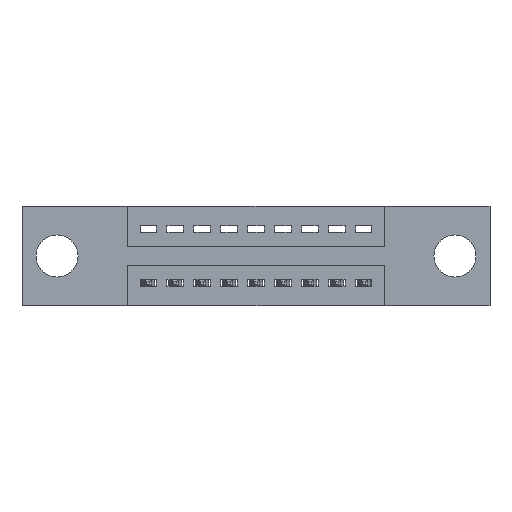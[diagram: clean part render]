
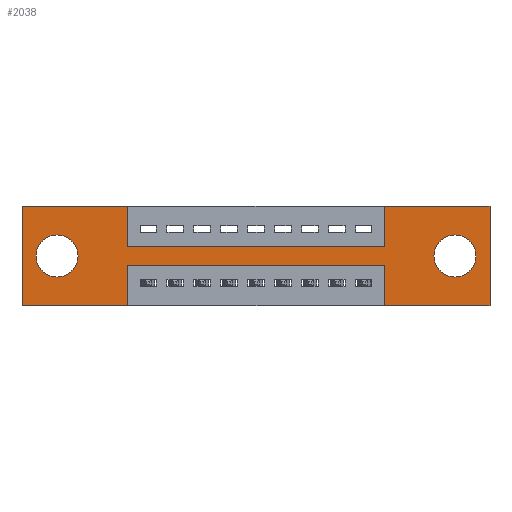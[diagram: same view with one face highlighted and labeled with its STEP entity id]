
A CAD part, front view. The second image highlights one B-rep face of the part: STEP entity #2038.
In plain terms, the highlighted planar face has unit normal (0, -1, 0).
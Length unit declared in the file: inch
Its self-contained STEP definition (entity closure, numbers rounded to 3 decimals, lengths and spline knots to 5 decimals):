
#24 = ORIENTED_EDGE ( 'NONE', *, *, #10581, .F. ) ;
#48 = DIRECTION ( 'NONE',  ( 0., 1., 0. ) ) ;
#113 = CARTESIAN_POINT ( 'NONE',  ( 0.13, 0., -0.185 ) ) ;
#126 = EDGE_LOOP ( 'NONE', ( #5890, #6085, #3829, #6019, #745, #6977, #2964, #5603, #10811, #10985, #5366, #24 ) ) ;
#154 = VECTOR ( 'NONE', #1543, 39.37008 ) ;
#226 = DIRECTION ( 'NONE',  ( 0., 1., 0. ) ) ;
#268 = CARTESIAN_POINT ( 'NONE',  ( 1.3425, 0., -0.15 ) ) ;
#337 = DIRECTION ( 'NONE',  ( 0., 0., -1. ) ) ;
#339 = CIRCLE ( 'NONE', #676, 0.078 ) ;
#390 = CARTESIAN_POINT ( 'NONE',  ( 0., 0., -0.37 ) ) ;
#392 = CIRCLE ( 'NONE', #1590, 0.078 ) ;
#396 = VERTEX_POINT ( 'NONE', #7209 ) ;
#422 = EDGE_CURVE ( 'NONE', #6330, #3517, #10646, .T. ) ;
#447 = CARTESIAN_POINT ( 'NONE',  ( 0.3925, 0., -0.22 ) ) ;
#501 = CARTESIAN_POINT ( 'NONE',  ( 1.605, 0., -0.263 ) ) ;
#584 = VECTOR ( 'NONE', #5580, 39.37008 ) ;
#661 = VECTOR ( 'NONE', #5711, 39.37008 ) ;
#672 = LINE ( 'NONE', #390, #9930 ) ;
#676 = AXIS2_PLACEMENT_3D ( 'NONE', #7832, #48, #2664 ) ;
#745 = ORIENTED_EDGE ( 'NONE', *, *, #4277, .F. ) ;
#799 = VERTEX_POINT ( 'NONE', #3179 ) ;
#807 = VERTEX_POINT ( 'NONE', #10939 ) ;
#849 = VECTOR ( 'NONE', #971, 39.37008 ) ;
#971 = DIRECTION ( 'NONE',  ( 0., 0., 1. ) ) ;
#1173 = CARTESIAN_POINT ( 'NONE',  ( 1.605, 0., -0.185 ) ) ;
#1176 = ORIENTED_EDGE ( 'NONE', *, *, #8504, .T. ) ;
#1543 = DIRECTION ( 'NONE',  ( -1., 0., 0. ) ) ;
#1576 = CARTESIAN_POINT ( 'NONE',  ( 1.735, 0., 0. ) ) ;
#1590 = AXIS2_PLACEMENT_3D ( 'NONE', #1173, #3766, #337 ) ;
#1688 = CARTESIAN_POINT ( 'NONE',  ( 0., 0., 0. ) ) ;
#1762 = CARTESIAN_POINT ( 'NONE',  ( 1.3425, 0., -0.22 ) ) ;
#2038 = ADVANCED_FACE ( 'NONE', ( #9285, #2340, #5317 ), #4694, .T. ) ;
#2233 = DIRECTION ( 'NONE',  ( 1., 0., 0. ) ) ;
#2272 = EDGE_CURVE ( 'NONE', #6221, #807, #6128, .T. ) ;
#2276 = DIRECTION ( 'NONE',  ( 0., 0., 1. ) ) ;
#2340 = FACE_BOUND ( 'NONE', #10150, .T. ) ;
#2423 = DIRECTION ( 'NONE',  ( 1., 0., 0. ) ) ;
#2607 = AXIS2_PLACEMENT_3D ( 'NONE', #6830, #6025, #8680 ) ;
#2634 = VERTEX_POINT ( 'NONE', #7970 ) ;
#2664 = DIRECTION ( 'NONE',  ( 0., 0., 1. ) ) ;
#2705 = CARTESIAN_POINT ( 'NONE',  ( 0.3925, 0., -0.22 ) ) ;
#2796 = CARTESIAN_POINT ( 'NONE',  ( 0., 0., 0. ) ) ;
#2964 = ORIENTED_EDGE ( 'NONE', *, *, #2272, .F. ) ;
#3005 = EDGE_CURVE ( 'NONE', #807, #10162, #8576, .T. ) ;
#3008 = DIRECTION ( 'NONE',  ( 0., 0., -1. ) ) ;
#3048 = LINE ( 'NONE', #2796, #8111 ) ;
#3080 = DIRECTION ( 'NONE',  ( 1., 0., 0. ) ) ;
#3179 = CARTESIAN_POINT ( 'NONE',  ( 0.13, 0., -0.107 ) ) ;
#3517 = VERTEX_POINT ( 'NONE', #1762 ) ;
#3636 = VERTEX_POINT ( 'NONE', #501 ) ;
#3766 = DIRECTION ( 'NONE',  ( 0., 1., 0. ) ) ;
#3829 = ORIENTED_EDGE ( 'NONE', *, *, #422, .F. ) ;
#3936 = VECTOR ( 'NONE', #2423, 39.37008 ) ;
#4048 = VERTEX_POINT ( 'NONE', #4956 ) ;
#4277 = EDGE_CURVE ( 'NONE', #10162, #396, #4987, .T. ) ;
#4488 = EDGE_CURVE ( 'NONE', #3636, #10643, #392, .T. ) ;
#4516 = DIRECTION ( 'NONE',  ( 0., 0., 1. ) ) ;
#4694 = PLANE ( 'NONE',  #7392 ) ;
#4696 = CARTESIAN_POINT ( 'NONE',  ( 1.605, 0., -0.107 ) ) ;
#4730 = EDGE_CURVE ( 'NONE', #10643, #3636, #4827, .T. ) ;
#4827 = CIRCLE ( 'NONE', #2607, 0.078 ) ;
#4946 = CARTESIAN_POINT ( 'NONE',  ( 1.3425, 0., 0. ) ) ;
#4947 = VERTEX_POINT ( 'NONE', #8941 ) ;
#4956 = CARTESIAN_POINT ( 'NONE',  ( 0., 0., 0. ) ) ;
#4987 = LINE ( 'NONE', #6201, #661 ) ;
#5139 = ORIENTED_EDGE ( 'NONE', *, *, #4730, .T. ) ;
#5153 = CARTESIAN_POINT ( 'NONE',  ( 0.13, 0., -0.263 ) ) ;
#5169 = EDGE_CURVE ( 'NONE', #2634, #4048, #3048, .T. ) ;
#5288 = LINE ( 'NONE', #7436, #10069 ) ;
#5317 = FACE_OUTER_BOUND ( 'NONE', #126, .T. ) ;
#5349 = VECTOR ( 'NONE', #2233, 39.37008 ) ;
#5366 = ORIENTED_EDGE ( 'NONE', *, *, #5169, .F. ) ;
#5531 = DIRECTION ( 'NONE',  ( 0., 0., -1. ) ) ;
#5580 = DIRECTION ( 'NONE',  ( -1., 0., 0. ) ) ;
#5603 = ORIENTED_EDGE ( 'NONE', *, *, #7728, .F. ) ;
#5608 = VECTOR ( 'NONE', #3008, 39.37008 ) ;
#5711 = DIRECTION ( 'NONE',  ( 0., 0., -1. ) ) ;
#5890 = ORIENTED_EDGE ( 'NONE', *, *, #7424, .F. ) ;
#5999 = EDGE_CURVE ( 'NONE', #8498, #799, #7178, .T. ) ;
#6019 = ORIENTED_EDGE ( 'NONE', *, *, #9727, .F. ) ;
#6025 = DIRECTION ( 'NONE',  ( 0., 1., 0. ) ) ;
#6085 = ORIENTED_EDGE ( 'NONE', *, *, #9084, .F. ) ;
#6128 = LINE ( 'NONE', #4946, #10776 ) ;
#6201 = CARTESIAN_POINT ( 'NONE',  ( 1.735, 0., 0. ) ) ;
#6221 = VERTEX_POINT ( 'NONE', #268 ) ;
#6263 = AXIS2_PLACEMENT_3D ( 'NONE', #113, #226, #4516 ) ;
#6330 = VERTEX_POINT ( 'NONE', #8382 ) ;
#6388 = DIRECTION ( 'NONE',  ( -1., 0., 0. ) ) ;
#6579 = ORIENTED_EDGE ( 'NONE', *, *, #4488, .T. ) ;
#6830 = CARTESIAN_POINT ( 'NONE',  ( 1.605, 0., -0.185 ) ) ;
#6977 = ORIENTED_EDGE ( 'NONE', *, *, #3005, .F. ) ;
#7178 = CIRCLE ( 'NONE', #6263, 0.078 ) ;
#7209 = CARTESIAN_POINT ( 'NONE',  ( 1.735, 0., -0.37 ) ) ;
#7272 = CARTESIAN_POINT ( 'NONE',  ( 0.3925, 0., -0.37 ) ) ;
#7360 = LINE ( 'NONE', #11218, #154 ) ;
#7392 = AXIS2_PLACEMENT_3D ( 'NONE', #10061, #8349, #9111 ) ;
#7424 = EDGE_CURVE ( 'NONE', #9404, #8290, #10554, .T. ) ;
#7425 = CARTESIAN_POINT ( 'NONE',  ( 0.3925, 0., 0. ) ) ;
#7434 = CARTESIAN_POINT ( 'NONE',  ( 0.3925, 0., -0.15 ) ) ;
#7436 = CARTESIAN_POINT ( 'NONE',  ( 0., 0., 0. ) ) ;
#7540 = EDGE_CURVE ( 'NONE', #4947, #8645, #10275, .T. ) ;
#7728 = EDGE_CURVE ( 'NONE', #8645, #6221, #9308, .T. ) ;
#7832 = CARTESIAN_POINT ( 'NONE',  ( 0.13, 0., -0.185 ) ) ;
#7929 = CARTESIAN_POINT ( 'NONE',  ( 1.3425, 0., -0.37 ) ) ;
#7950 = VECTOR ( 'NONE', #5531, 39.37008 ) ;
#7970 = CARTESIAN_POINT ( 'NONE',  ( 0., 0., -0.37 ) ) ;
#8111 = VECTOR ( 'NONE', #9768, 39.37008 ) ;
#8290 = VERTEX_POINT ( 'NONE', #7272 ) ;
#8349 = DIRECTION ( 'NONE',  ( 0., -1., 0. ) ) ;
#8382 = CARTESIAN_POINT ( 'NONE',  ( 1.3425, 0., -0.37 ) ) ;
#8498 = VERTEX_POINT ( 'NONE', #5153 ) ;
#8504 = EDGE_CURVE ( 'NONE', #799, #8498, #339, .T. ) ;
#8576 = LINE ( 'NONE', #1688, #3936 ) ;
#8645 = VERTEX_POINT ( 'NONE', #9783 ) ;
#8680 = DIRECTION ( 'NONE',  ( 0., 0., -1. ) ) ;
#8941 = CARTESIAN_POINT ( 'NONE',  ( 0.3925, 0., 0. ) ) ;
#9084 = EDGE_CURVE ( 'NONE', #3517, #9404, #10651, .T. ) ;
#9111 = DIRECTION ( 'NONE',  ( 0., 0., -1. ) ) ;
#9285 = FACE_BOUND ( 'NONE', #10358, .T. ) ;
#9308 = LINE ( 'NONE', #7434, #5349 ) ;
#9404 = VERTEX_POINT ( 'NONE', #447 ) ;
#9727 = EDGE_CURVE ( 'NONE', #396, #6330, #7360, .T. ) ;
#9768 = DIRECTION ( 'NONE',  ( 0., 0., 1. ) ) ;
#9774 = ORIENTED_EDGE ( 'NONE', *, *, #5999, .T. ) ;
#9783 = CARTESIAN_POINT ( 'NONE',  ( 0.3925, 0., -0.15 ) ) ;
#9819 = CARTESIAN_POINT ( 'NONE',  ( 0.3925, 0., -0.37 ) ) ;
#9930 = VECTOR ( 'NONE', #6388, 39.37008 ) ;
#10061 = CARTESIAN_POINT ( 'NONE',  ( 0., 0., -0.37 ) ) ;
#10069 = VECTOR ( 'NONE', #3080, 39.37008 ) ;
#10150 = EDGE_LOOP ( 'NONE', ( #1176, #9774 ) ) ;
#10162 = VERTEX_POINT ( 'NONE', #1576 ) ;
#10219 = EDGE_CURVE ( 'NONE', #4048, #4947, #5288, .T. ) ;
#10275 = LINE ( 'NONE', #7425, #5608 ) ;
#10358 = EDGE_LOOP ( 'NONE', ( #5139, #6579 ) ) ;
#10554 = LINE ( 'NONE', #9819, #7950 ) ;
#10581 = EDGE_CURVE ( 'NONE', #8290, #2634, #672, .T. ) ;
#10643 = VERTEX_POINT ( 'NONE', #4696 ) ;
#10646 = LINE ( 'NONE', #7929, #849 ) ;
#10651 = LINE ( 'NONE', #2705, #584 ) ;
#10776 = VECTOR ( 'NONE', #2276, 39.37008 ) ;
#10811 = ORIENTED_EDGE ( 'NONE', *, *, #7540, .F. ) ;
#10939 = CARTESIAN_POINT ( 'NONE',  ( 1.3425, 0., 0. ) ) ;
#10985 = ORIENTED_EDGE ( 'NONE', *, *, #10219, .F. ) ;
#11218 = CARTESIAN_POINT ( 'NONE',  ( 0., 0., -0.37 ) ) ;
